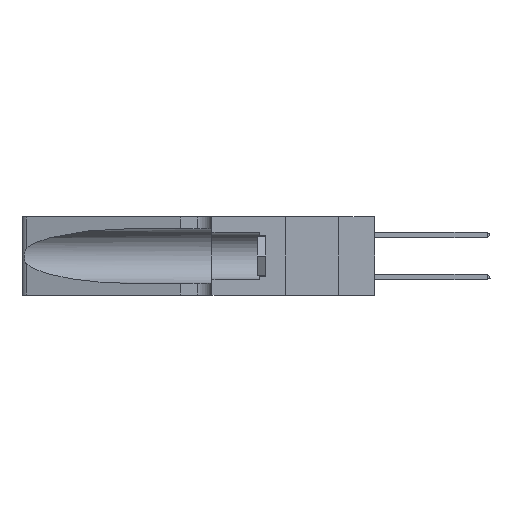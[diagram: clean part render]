
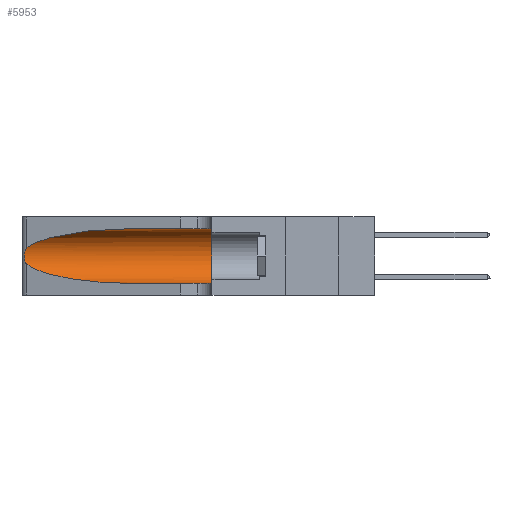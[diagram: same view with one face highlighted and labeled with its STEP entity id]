
A CAD part, left-side view. The second image highlights one B-rep face of the part: STEP entity #5953.
In plain terms, the highlighted cylindrical face has radius 3.308 mm (diameter 6.617 mm), a partial arc.
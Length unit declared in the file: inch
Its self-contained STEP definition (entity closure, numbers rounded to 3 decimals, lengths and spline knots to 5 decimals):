
#520 = CARTESIAN_POINT ( 'NONE',  ( 0.2373, 1.15595, 0.28018 ) ) ;
#539 = CARTESIAN_POINT ( 'NONE',  ( 0.1305, 1.61858, 0.05475 ) ) ;
#744 = CARTESIAN_POINT ( 'NONE',  ( 0.25555, 1.22993, 0.14849 ) ) ;
#1671 = CARTESIAN_POINT ( 'NONE',  ( 0.2373, 1.15595, 0.08982 ) ) ;
#2014 =( BOUNDED_CURVE ( )  B_SPLINE_CURVE ( 3, ( #22687, #10850, #520, #15903 ),
 .UNSPECIFIED., .F., .F. ) 
 B_SPLINE_CURVE_WITH_KNOTS ( ( 4, 4 ),
 ( 1.5708, 2.84003 ),
 .UNSPECIFIED. ) 
 CURVE ( )  GEOMETRIC_REPRESENTATION_ITEM ( )  RATIONAL_B_SPLINE_CURVE ( ( 1., 0.87, 0.87, 1. ) ) 
 REPRESENTATION_ITEM ( '' )  );
#2299 = DIRECTION ( 'NONE',  ( 0., -1., 0. ) ) ;
#2531 = CARTESIAN_POINT ( 'NONE',  ( 0.26075, 1.23896, 0.19203 ) ) ;
#2787 = EDGE_CURVE ( 'NONE', #16622, #8168, #3653, .T. ) ;
#3177 = EDGE_CURVE ( 'NONE', #8168, #32565, #12816, .T. ) ;
#3400 = CARTESIAN_POINT ( 'NONE',  ( 0.25487, 1.22718, 0.14631 ) ) ;
#3653 = B_SPLINE_CURVE_WITH_KNOTS ( 'NONE', 3,
 ( #7957, #32663, #15159, #5030, #7742, #27877, #2531, #13292, #25997, #5520, #26103, #25890, #744, #3400 ),
 .UNSPECIFIED., .F., .F.,
 ( 4, 2, 2, 2, 2, 2, 4 ),
 ( 0., 0.00027, 0.00053, 0.00107, 0.0016, 0.00187, 0.00214 ),
 .UNSPECIFIED. ) ;
#4704 = VERTEX_POINT ( 'NONE', #18028 ) ;
#4707 = EDGE_CURVE ( 'NONE', #20840, #4704, #31879, .T. ) ;
#4828 = EDGE_CURVE ( 'NONE', #8300, #16622, #2014, .T. ) ;
#5030 = CARTESIAN_POINT ( 'NONE',  ( 0.25787, 1.23484, 0.2124 ) ) ;
#5520 = CARTESIAN_POINT ( 'NONE',  ( 0.25856, 1.23593, 0.16098 ) ) ;
#5646 = ORIENTED_EDGE ( 'NONE', *, *, #4707, .F. ) ;
#5953 = ADVANCED_FACE ( 'NONE', ( #31434 ), #6567, .F. ) ;
#6567 = CYLINDRICAL_SURFACE ( 'NONE', #8235, 0.13025 ) ;
#7152 = ORIENTED_EDGE ( 'NONE', *, *, #27943, .T. ) ;
#7742 = CARTESIAN_POINT ( 'NONE',  ( 0.25854, 1.2359, 0.20912 ) ) ;
#7957 = CARTESIAN_POINT ( 'NONE',  ( 0.25487, 1.22718, 0.22369 ) ) ;
#8168 = VERTEX_POINT ( 'NONE', #13738 ) ;
#8235 = AXIS2_PLACEMENT_3D ( 'NONE', #9849, #2299, #9970 ) ;
#8300 = VERTEX_POINT ( 'NONE', #19188 ) ;
#9849 = CARTESIAN_POINT ( 'NONE',  ( 0.1305, 1.61858, 0.185 ) ) ;
#9970 = DIRECTION ( 'NONE',  ( 0., 0., -1. ) ) ;
#10850 = CARTESIAN_POINT ( 'NONE',  ( 0.18966, 0.96281, 0.31525 ) ) ;
#12037 = VECTOR ( 'NONE', #16690, 39.37008 ) ;
#12217 = CARTESIAN_POINT ( 'NONE',  ( 0.1305, 0.35, 0.31525 ) ) ;
#12591 = LINE ( 'NONE', #539, #30301 ) ;
#12816 =( BOUNDED_CURVE ( )  B_SPLINE_CURVE ( 3, ( #26486, #1671, #19264, #18920 ),
 .UNSPECIFIED., .F., .T. ) 
 B_SPLINE_CURVE_WITH_KNOTS ( ( 4, 4 ),
 ( 3.44316, 4.71239 ),
 .UNSPECIFIED. ) 
 CURVE ( )  GEOMETRIC_REPRESENTATION_ITEM ( )  RATIONAL_B_SPLINE_CURVE ( ( 1., 0.87, 0.87, 1. ) ) 
 REPRESENTATION_ITEM ( '' )  );
#12834 = CARTESIAN_POINT ( 'NONE',  ( 0.1305, 0.35, 0.185 ) ) ;
#13292 = CARTESIAN_POINT ( 'NONE',  ( 0.26075, 1.23896, 0.178 ) ) ;
#13738 = CARTESIAN_POINT ( 'NONE',  ( 0.25487, 1.22718, 0.14631 ) ) ;
#14260 = CARTESIAN_POINT ( 'NONE',  ( 0.1305, 0.72297, 0.05475 ) ) ;
#14529 = ORIENTED_EDGE ( 'NONE', *, *, #2787, .T. ) ;
#15159 = CARTESIAN_POINT ( 'NONE',  ( 0.25639, 1.23184, 0.21858 ) ) ;
#15903 = CARTESIAN_POINT ( 'NONE',  ( 0.25487, 1.22718, 0.22369 ) ) ;
#16622 = VERTEX_POINT ( 'NONE', #29472 ) ;
#16690 = DIRECTION ( 'NONE',  ( 0., -1., 0. ) ) ;
#17481 = AXIS2_PLACEMENT_3D ( 'NONE', #12834, #32659, #30225 ) ;
#18028 = CARTESIAN_POINT ( 'NONE',  ( 0.1305, 0.35, 0.05475 ) ) ;
#18920 = CARTESIAN_POINT ( 'NONE',  ( 0.1305, 0.72297, 0.05475 ) ) ;
#19188 = CARTESIAN_POINT ( 'NONE',  ( 0.1305, 0.72297, 0.31525 ) ) ;
#19264 = CARTESIAN_POINT ( 'NONE',  ( 0.18966, 0.96281, 0.05475 ) ) ;
#20840 = VERTEX_POINT ( 'NONE', #12217 ) ;
#21445 = LINE ( 'NONE', #31798, #12037 ) ;
#22329 = ORIENTED_EDGE ( 'NONE', *, *, #4828, .T. ) ;
#22687 = CARTESIAN_POINT ( 'NONE',  ( 0.1305, 0.72297, 0.31525 ) ) ;
#25479 = ORIENTED_EDGE ( 'NONE', *, *, #30867, .F. ) ;
#25890 = CARTESIAN_POINT ( 'NONE',  ( 0.25639, 1.23186, 0.15144 ) ) ;
#25997 = CARTESIAN_POINT ( 'NONE',  ( 0.26017, 1.23833, 0.17102 ) ) ;
#26103 = CARTESIAN_POINT ( 'NONE',  ( 0.25789, 1.23486, 0.15765 ) ) ;
#26486 = CARTESIAN_POINT ( 'NONE',  ( 0.25487, 1.22718, 0.14631 ) ) ;
#27115 = ORIENTED_EDGE ( 'NONE', *, *, #3177, .T. ) ;
#27877 = CARTESIAN_POINT ( 'NONE',  ( 0.26018, 1.23835, 0.19895 ) ) ;
#27943 = EDGE_CURVE ( 'NONE', #32565, #4704, #12591, .T. ) ;
#29472 = CARTESIAN_POINT ( 'NONE',  ( 0.25487, 1.22718, 0.22369 ) ) ;
#30225 = DIRECTION ( 'NONE',  ( 0., 0., 1. ) ) ;
#30301 = VECTOR ( 'NONE', #30892, 39.37008 ) ;
#30377 = EDGE_LOOP ( 'NONE', ( #22329, #14529, #27115, #7152, #5646, #25479 ) ) ;
#30867 = EDGE_CURVE ( 'NONE', #8300, #20840, #21445, .T. ) ;
#30892 = DIRECTION ( 'NONE',  ( 0., -1., 0. ) ) ;
#31434 = FACE_OUTER_BOUND ( 'NONE', #30377, .T. ) ;
#31798 = CARTESIAN_POINT ( 'NONE',  ( 0.1305, 1.61858, 0.31525 ) ) ;
#31879 = CIRCLE ( 'NONE', #17481, 0.13025 ) ;
#32565 = VERTEX_POINT ( 'NONE', #14260 ) ;
#32659 = DIRECTION ( 'NONE',  ( 0., 1., 0. ) ) ;
#32663 = CARTESIAN_POINT ( 'NONE',  ( 0.25555, 1.22994, 0.2215 ) ) ;
